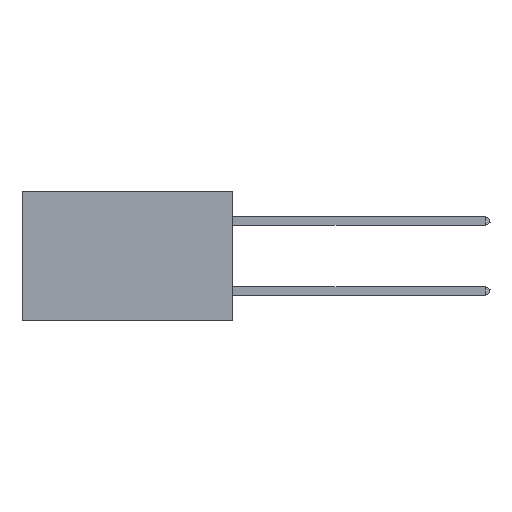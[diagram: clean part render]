
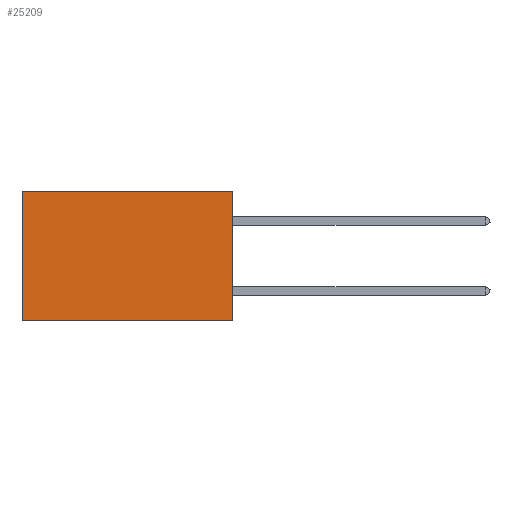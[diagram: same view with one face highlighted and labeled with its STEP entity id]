
A CAD part, left-side view. The second image highlights one B-rep face of the part: STEP entity #25209.
In plain terms, the highlighted planar face has unit normal (-1, 0, 0).
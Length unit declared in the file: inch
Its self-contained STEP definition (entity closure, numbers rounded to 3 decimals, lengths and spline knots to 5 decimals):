
#459 = CARTESIAN_POINT ( 'NONE',  ( 0.2875, 0.6, -0.37 ) ) ;
#1820 = DIRECTION ( 'NONE',  ( 0., 0., -1. ) ) ;
#1912 = ORIENTED_EDGE ( 'NONE', *, *, #28186, .F. ) ;
#2585 = DIRECTION ( 'NONE',  ( 0., 0., -1. ) ) ;
#2995 = LINE ( 'NONE', #22506, #15454 ) ;
#4446 = AXIS2_PLACEMENT_3D ( 'NONE', #8824, #13810, #30965 ) ;
#4711 = DIRECTION ( 'NONE',  ( 0., 1., 0. ) ) ;
#6797 = VERTEX_POINT ( 'NONE', #14580 ) ;
#8163 = VERTEX_POINT ( 'NONE', #18920 ) ;
#8824 = CARTESIAN_POINT ( 'NONE',  ( 0.2875, 0., 0. ) ) ;
#9119 = LINE ( 'NONE', #31295, #21546 ) ;
#10040 = ORIENTED_EDGE ( 'NONE', *, *, #17699, .F. ) ;
#11168 = EDGE_CURVE ( 'NONE', #8163, #16753, #9119, .T. ) ;
#11590 = ORIENTED_EDGE ( 'NONE', *, *, #11168, .T. ) ;
#12051 = FACE_OUTER_BOUND ( 'NONE', #22975, .T. ) ;
#13276 = VECTOR ( 'NONE', #16343, 39.37008 ) ;
#13810 = DIRECTION ( 'NONE',  ( 1., 0., 0. ) ) ;
#13811 = CARTESIAN_POINT ( 'NONE',  ( 0.2875, 0., -0.37 ) ) ;
#14580 = CARTESIAN_POINT ( 'NONE',  ( 0.2875, 0., -0.37 ) ) ;
#15066 = VECTOR ( 'NONE', #4711, 39.37008 ) ;
#15454 = VECTOR ( 'NONE', #2585, 39.37008 ) ;
#16343 = DIRECTION ( 'NONE',  ( 0., 1., 0. ) ) ;
#16753 = VERTEX_POINT ( 'NONE', #459 ) ;
#17699 = EDGE_CURVE ( 'NONE', #6797, #16753, #27145, .T. ) ;
#18920 = CARTESIAN_POINT ( 'NONE',  ( 0.2875, 0.6, 0. ) ) ;
#20763 = EDGE_CURVE ( 'NONE', #29436, #8163, #21617, .T. ) ;
#21546 = VECTOR ( 'NONE', #1820, 39.37008 ) ;
#21617 = LINE ( 'NONE', #26824, #15066 ) ;
#22506 = CARTESIAN_POINT ( 'NONE',  ( 0.2875, 0., 0. ) ) ;
#22975 = EDGE_LOOP ( 'NONE', ( #11590, #10040, #1912, #31745 ) ) ;
#23339 = CARTESIAN_POINT ( 'NONE',  ( 0.2875, 0., 0. ) ) ;
#25209 = ADVANCED_FACE ( 'NONE', ( #12051 ), #26102, .F. ) ;
#26102 = PLANE ( 'NONE',  #4446 ) ;
#26824 = CARTESIAN_POINT ( 'NONE',  ( 0.2875, 0., 0. ) ) ;
#27145 = LINE ( 'NONE', #13811, #13276 ) ;
#28186 = EDGE_CURVE ( 'NONE', #29436, #6797, #2995, .T. ) ;
#29436 = VERTEX_POINT ( 'NONE', #23339 ) ;
#30965 = DIRECTION ( 'NONE',  ( 0., 0., -1. ) ) ;
#31295 = CARTESIAN_POINT ( 'NONE',  ( 0.2875, 0.6, 0. ) ) ;
#31745 = ORIENTED_EDGE ( 'NONE', *, *, #20763, .T. ) ;
